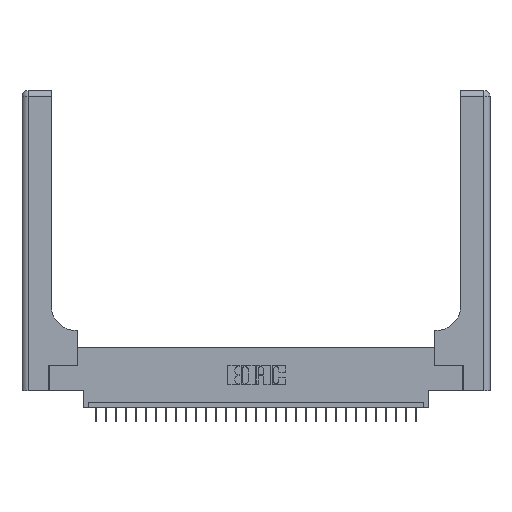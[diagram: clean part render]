
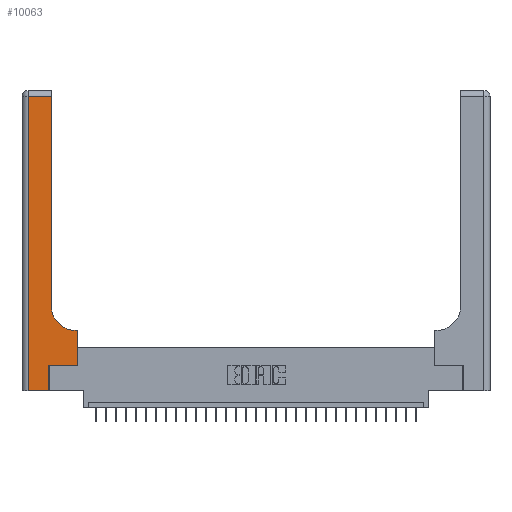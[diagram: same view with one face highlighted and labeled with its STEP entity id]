
A CAD part, top view. The second image highlights one B-rep face of the part: STEP entity #10063.
In plain terms, the highlighted planar face has unit normal (0, 0, 1).
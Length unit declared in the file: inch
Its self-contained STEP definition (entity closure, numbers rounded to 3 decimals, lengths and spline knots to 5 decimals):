
#3168 = VECTOR ( 'NONE', #29179, 39.37008 ) ;
#3189 = EDGE_CURVE ( 'NONE', #3235, #19132, #24788, .T. ) ;
#3235 = VERTEX_POINT ( 'NONE', #28405 ) ;
#3497 = CARTESIAN_POINT ( 'NONE',  ( 0.5585, 0.6, 0.37 ) ) ;
#3515 = CARTESIAN_POINT ( 'NONE',  ( 0.5415, 0.85, 0.37 ) ) ;
#3588 = LINE ( 'NONE', #10609, #10819 ) ;
#3713 = LINE ( 'NONE', #18999, #15126 ) ;
#3824 = DIRECTION ( 'NONE',  ( 0., -1., 0. ) ) ;
#4963 = LINE ( 'NONE', #23047, #12215 ) ;
#5571 = PLANE ( 'NONE',  #28845 ) ;
#7625 = ORIENTED_EDGE ( 'NONE', *, *, #29067, .T. ) ;
#7931 = ORIENTED_EDGE ( 'NONE', *, *, #14152, .T. ) ;
#8380 = ORIENTED_EDGE ( 'NONE', *, *, #15502, .T. ) ;
#8383 = DIRECTION ( 'NONE',  ( -1., 0., 0. ) ) ;
#8677 = EDGE_CURVE ( 'NONE', #16319, #9521, #3713, .T. ) ;
#9014 = VERTEX_POINT ( 'NONE', #22807 ) ;
#9222 = LINE ( 'NONE', #28324, #15672 ) ;
#9521 = VERTEX_POINT ( 'NONE', #29460 ) ;
#10063 = ADVANCED_FACE ( 'NONE', ( #27525 ), #5571, .F. ) ;
#10512 = VECTOR ( 'NONE', #27706, 39.37008 ) ;
#10533 = CARTESIAN_POINT ( 'NONE',  ( 0.269, 0., 0.37 ) ) ;
#10606 = CARTESIAN_POINT ( 'NONE',  ( 0.269, 0., 0.37 ) ) ;
#10609 = CARTESIAN_POINT ( 'NONE',  ( 0.2915, 0.6, 0.37 ) ) ;
#10710 = CARTESIAN_POINT ( 'NONE',  ( 0.06, 0., 0.37 ) ) ;
#10819 = VECTOR ( 'NONE', #8383, 39.37008 ) ;
#11519 = DIRECTION ( 'NONE',  ( -1., 0., 0. ) ) ;
#12148 = VERTEX_POINT ( 'NONE', #29504 ) ;
#12215 = VECTOR ( 'NONE', #25137, 39.37008 ) ;
#12606 = LINE ( 'NONE', #20385, #10512 ) ;
#12686 = CARTESIAN_POINT ( 'NONE',  ( 0.5585, 0.25, 0.37 ) ) ;
#13334 = ORIENTED_EDGE ( 'NONE', *, *, #20768, .T. ) ;
#13609 = VECTOR ( 'NONE', #20085, 39.37008 ) ;
#13890 = AXIS2_PLACEMENT_3D ( 'NONE', #3515, #21189, #27716 ) ;
#14029 = EDGE_LOOP ( 'NONE', ( #7931, #17380, #23758, #7625, #8380, #13334, #27987, #31014, #17372 ) ) ;
#14152 = EDGE_CURVE ( 'NONE', #15574, #16319, #12606, .T. ) ;
#14883 = CARTESIAN_POINT ( 'NONE',  ( 0., 0., 0.37 ) ) ;
#15126 = VECTOR ( 'NONE', #11519, 39.37008 ) ;
#15502 = EDGE_CURVE ( 'NONE', #16454, #9014, #18176, .T. ) ;
#15574 = VERTEX_POINT ( 'NONE', #27399 ) ;
#15666 = EDGE_CURVE ( 'NONE', #9521, #20614, #9222, .T. ) ;
#15672 = VECTOR ( 'NONE', #3824, 39.37008 ) ;
#16319 = VERTEX_POINT ( 'NONE', #31279 ) ;
#16454 = VERTEX_POINT ( 'NONE', #10606 ) ;
#17372 = ORIENTED_EDGE ( 'NONE', *, *, #29476, .T. ) ;
#17380 = ORIENTED_EDGE ( 'NONE', *, *, #8677, .T. ) ;
#17431 = LINE ( 'NONE', #14883, #3168 ) ;
#18176 = LINE ( 'NONE', #10533, #13609 ) ;
#18999 = CARTESIAN_POINT ( 'NONE',  ( 0., 2.94, 0.37 ) ) ;
#19132 = VERTEX_POINT ( 'NONE', #3497 ) ;
#20085 = DIRECTION ( 'NONE',  ( 0., 1., 0. ) ) ;
#20218 = DIRECTION ( 'NONE',  ( 0., 0., -1. ) ) ;
#20385 = CARTESIAN_POINT ( 'NONE',  ( 0.2915, 3., 0.37 ) ) ;
#20526 = DIRECTION ( 'NONE',  ( -1., 0., 0. ) ) ;
#20614 = VERTEX_POINT ( 'NONE', #10710 ) ;
#20768 = EDGE_CURVE ( 'NONE', #9014, #3235, #4963, .T. ) ;
#21189 = DIRECTION ( 'NONE',  ( 0., 0., -1. ) ) ;
#22807 = CARTESIAN_POINT ( 'NONE',  ( 0.269, 0.25, 0.37 ) ) ;
#23047 = CARTESIAN_POINT ( 'NONE',  ( 0.269, 0.25, 0.37 ) ) ;
#23758 = ORIENTED_EDGE ( 'NONE', *, *, #15666, .T. ) ;
#24788 = LINE ( 'NONE', #12686, #29124 ) ;
#25137 = DIRECTION ( 'NONE',  ( 1., 0., 0. ) ) ;
#25570 = CIRCLE ( 'NONE', #13890, 0.25 ) ;
#27320 = DIRECTION ( 'NONE',  ( 0., 1., 0. ) ) ;
#27399 = CARTESIAN_POINT ( 'NONE',  ( 0.2915, 0.85, 0.37 ) ) ;
#27525 = FACE_OUTER_BOUND ( 'NONE', #14029, .T. ) ;
#27706 = DIRECTION ( 'NONE',  ( 0., 1., 0. ) ) ;
#27716 = DIRECTION ( 'NONE',  ( 1., 0., 0. ) ) ;
#27842 = CARTESIAN_POINT ( 'NONE',  ( 0., 3., 0.37 ) ) ;
#27987 = ORIENTED_EDGE ( 'NONE', *, *, #3189, .T. ) ;
#28324 = CARTESIAN_POINT ( 'NONE',  ( 0.06, 3., 0.37 ) ) ;
#28405 = CARTESIAN_POINT ( 'NONE',  ( 0.5585, 0.25, 0.37 ) ) ;
#28842 = EDGE_CURVE ( 'NONE', #19132, #12148, #3588, .T. ) ;
#28845 = AXIS2_PLACEMENT_3D ( 'NONE', #27842, #20218, #20526 ) ;
#29067 = EDGE_CURVE ( 'NONE', #20614, #16454, #17431, .T. ) ;
#29124 = VECTOR ( 'NONE', #27320, 39.37008 ) ;
#29179 = DIRECTION ( 'NONE',  ( 1., 0., 0. ) ) ;
#29460 = CARTESIAN_POINT ( 'NONE',  ( 0.06, 2.94, 0.37 ) ) ;
#29476 = EDGE_CURVE ( 'NONE', #12148, #15574, #25570, .T. ) ;
#29504 = CARTESIAN_POINT ( 'NONE',  ( 0.5415, 0.6, 0.37 ) ) ;
#31014 = ORIENTED_EDGE ( 'NONE', *, *, #28842, .T. ) ;
#31279 = CARTESIAN_POINT ( 'NONE',  ( 0.2915, 2.94, 0.37 ) ) ;
